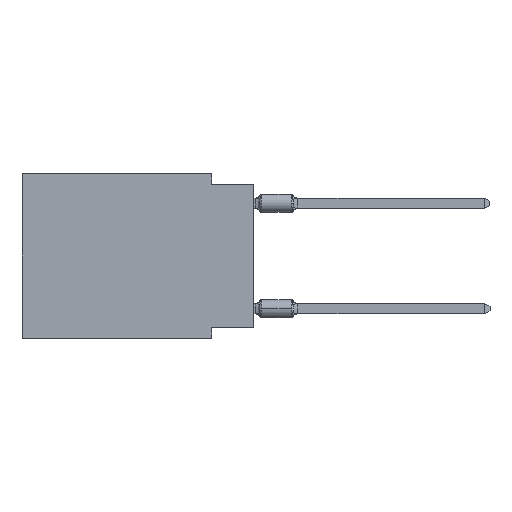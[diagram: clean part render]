
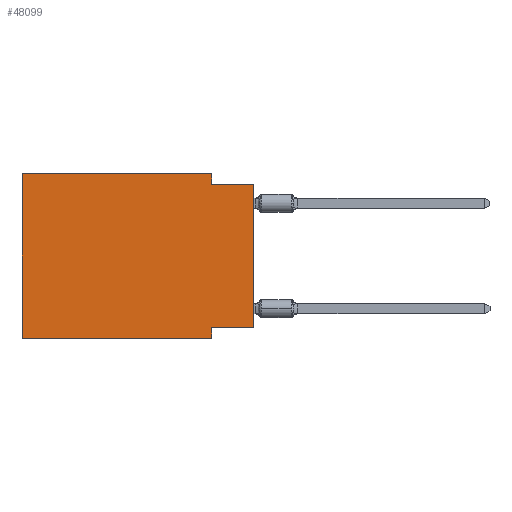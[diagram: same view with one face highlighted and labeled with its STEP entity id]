
A CAD part, left-side view. The second image highlights one B-rep face of the part: STEP entity #48099.
In plain terms, the highlighted planar face has unit normal (-1, 0, 0).
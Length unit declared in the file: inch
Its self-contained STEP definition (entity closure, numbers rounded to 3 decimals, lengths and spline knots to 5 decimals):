
#33 = VECTOR ( 'NONE', #2412, 39.37008 ) ;
#1329 = VECTOR ( 'NONE', #40849, 39.37008 ) ;
#1403 = ORIENTED_EDGE ( 'NONE', *, *, #30913, .F. ) ;
#2347 = EDGE_CURVE ( 'NONE', #2491, #28164, #7690, .T. ) ;
#2412 = DIRECTION ( 'NONE',  ( 0., -1., 0. ) ) ;
#2491 = VERTEX_POINT ( 'NONE', #46648 ) ;
#3910 = CARTESIAN_POINT ( 'NONE',  ( 0., 0., 0. ) ) ;
#4336 = DIRECTION ( 'NONE',  ( 1., 0., 0. ) ) ;
#5747 = CARTESIAN_POINT ( 'NONE',  ( 0., 0.55, -0.39 ) ) ;
#6117 = CARTESIAN_POINT ( 'NONE',  ( 0., 0.55, 0. ) ) ;
#6186 = CARTESIAN_POINT ( 'NONE',  ( 0., 0.55, -0.39 ) ) ;
#7690 = LINE ( 'NONE', #26668, #37832 ) ;
#7781 = CARTESIAN_POINT ( 'NONE',  ( 0., 0.1, 0. ) ) ;
#9925 = EDGE_CURVE ( 'NONE', #34283, #28164, #16908, .T. ) ;
#11412 = LINE ( 'NONE', #3910, #35274 ) ;
#12809 = EDGE_CURVE ( 'NONE', #47529, #19534, #48111, .T. ) ;
#13120 = CARTESIAN_POINT ( 'NONE',  ( 0., 0., -0.365 ) ) ;
#14941 = EDGE_LOOP ( 'NONE', ( #28186, #48379, #41370, #33816, #1403, #47251, #16394, #17433 ) ) ;
#16394 = ORIENTED_EDGE ( 'NONE', *, *, #2347, .F. ) ;
#16908 = LINE ( 'NONE', #6186, #33 ) ;
#17433 = ORIENTED_EDGE ( 'NONE', *, *, #30092, .F. ) ;
#17745 = CARTESIAN_POINT ( 'NONE',  ( 0., 0.55, 0. ) ) ;
#17793 = VERTEX_POINT ( 'NONE', #17745 ) ;
#17863 = CARTESIAN_POINT ( 'NONE',  ( 0., 0., -0.025 ) ) ;
#18312 = LINE ( 'NONE', #6117, #36243 ) ;
#19149 = DIRECTION ( 'NONE',  ( 0., 0., 1. ) ) ;
#19534 = VERTEX_POINT ( 'NONE', #38565 ) ;
#19819 = CARTESIAN_POINT ( 'NONE',  ( 0., 0.55, 0. ) ) ;
#21501 = DIRECTION ( 'NONE',  ( 0., 1., 0. ) ) ;
#22060 = DIRECTION ( 'NONE',  ( 0., 0., 1. ) ) ;
#26668 = CARTESIAN_POINT ( 'NONE',  ( 0., 0.1, -0.39 ) ) ;
#26833 = FACE_OUTER_BOUND ( 'NONE', #14941, .T. ) ;
#27058 = LINE ( 'NONE', #41566, #36142 ) ;
#28018 = EDGE_CURVE ( 'NONE', #36509, #28200, #11412, .T. ) ;
#28164 = VERTEX_POINT ( 'NONE', #35416 ) ;
#28186 = ORIENTED_EDGE ( 'NONE', *, *, #28018, .T. ) ;
#28200 = VERTEX_POINT ( 'NONE', #17863 ) ;
#29035 = LINE ( 'NONE', #44285, #33009 ) ;
#29723 = EDGE_CURVE ( 'NONE', #17793, #47529, #27058, .T. ) ;
#30092 = EDGE_CURVE ( 'NONE', #36509, #2491, #29035, .T. ) ;
#30606 = DIRECTION ( 'NONE',  ( 0., 0., -1. ) ) ;
#30913 = EDGE_CURVE ( 'NONE', #34283, #17793, #18312, .T. ) ;
#32396 = LINE ( 'NONE', #48630, #37768 ) ;
#33009 = VECTOR ( 'NONE', #21501, 39.37008 ) ;
#33816 = ORIENTED_EDGE ( 'NONE', *, *, #29723, .F. ) ;
#34283 = VERTEX_POINT ( 'NONE', #5747 ) ;
#34836 = PLANE ( 'NONE',  #38994 ) ;
#35274 = VECTOR ( 'NONE', #19149, 39.37008 ) ;
#35416 = CARTESIAN_POINT ( 'NONE',  ( 0., 0.1, -0.39 ) ) ;
#36142 = VECTOR ( 'NONE', #49309, 39.37008 ) ;
#36243 = VECTOR ( 'NONE', #22060, 39.37008 ) ;
#36509 = VERTEX_POINT ( 'NONE', #13120 ) ;
#37768 = VECTOR ( 'NONE', #40895, 39.37008 ) ;
#37832 = VECTOR ( 'NONE', #39165, 39.37008 ) ;
#38565 = CARTESIAN_POINT ( 'NONE',  ( 0., 0.1, -0.025 ) ) ;
#38994 = AXIS2_PLACEMENT_3D ( 'NONE', #19819, #4336, #30606 ) ;
#39165 = DIRECTION ( 'NONE',  ( 0., 0., -1. ) ) ;
#40440 = EDGE_CURVE ( 'NONE', #19534, #28200, #32396, .T. ) ;
#40849 = DIRECTION ( 'NONE',  ( 0., 0., -1. ) ) ;
#40895 = DIRECTION ( 'NONE',  ( 0., -1., 0. ) ) ;
#41370 = ORIENTED_EDGE ( 'NONE', *, *, #12809, .F. ) ;
#41566 = CARTESIAN_POINT ( 'NONE',  ( 0., 0.55, 0. ) ) ;
#44285 = CARTESIAN_POINT ( 'NONE',  ( 0., 0., -0.365 ) ) ;
#46546 = CARTESIAN_POINT ( 'NONE',  ( 0., 0.1, 0. ) ) ;
#46648 = CARTESIAN_POINT ( 'NONE',  ( 0., 0.1, -0.365 ) ) ;
#47251 = ORIENTED_EDGE ( 'NONE', *, *, #9925, .T. ) ;
#47529 = VERTEX_POINT ( 'NONE', #46546 ) ;
#48099 = ADVANCED_FACE ( 'NONE', ( #26833 ), #34836, .F. ) ;
#48111 = LINE ( 'NONE', #7781, #1329 ) ;
#48379 = ORIENTED_EDGE ( 'NONE', *, *, #40440, .F. ) ;
#48630 = CARTESIAN_POINT ( 'NONE',  ( 0., 0., -0.025 ) ) ;
#49309 = DIRECTION ( 'NONE',  ( 0., -1., 0. ) ) ;
